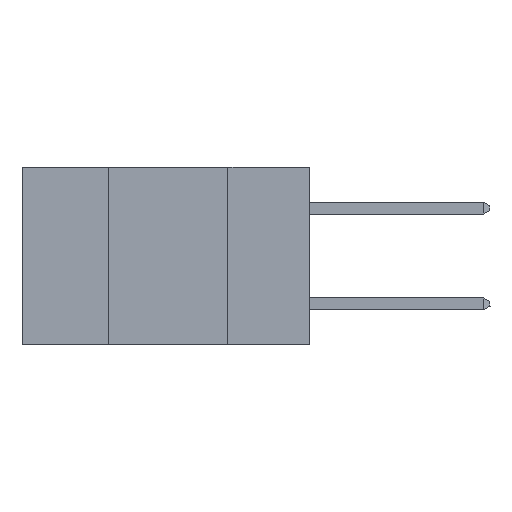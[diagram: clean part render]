
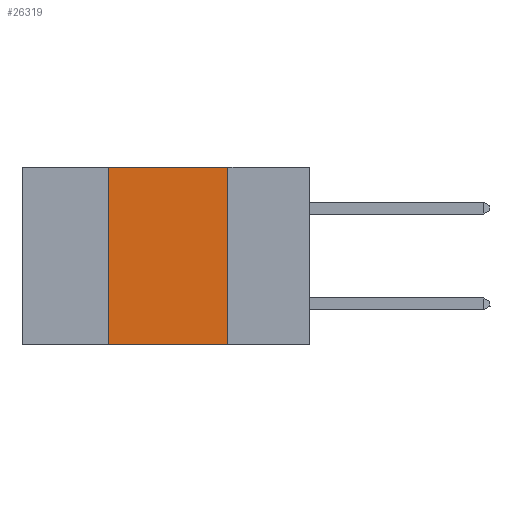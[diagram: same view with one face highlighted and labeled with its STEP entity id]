
A CAD part, left-side view. The second image highlights one B-rep face of the part: STEP entity #26319.
In plain terms, the highlighted planar face has unit normal (-1, 0, 0).
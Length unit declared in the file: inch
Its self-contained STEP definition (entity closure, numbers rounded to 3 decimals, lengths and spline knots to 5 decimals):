
#11 = CARTESIAN_POINT ( 'NONE',  ( 0., 0.6, -0.37 ) ) ;
#2732 = VERTEX_POINT ( 'NONE', #9013 ) ;
#4602 = LINE ( 'NONE', #24986, #17023 ) ;
#6655 = ORIENTED_EDGE ( 'NONE', *, *, #7911, .F. ) ;
#7911 = EDGE_CURVE ( 'NONE', #21412, #14088, #4602, .T. ) ;
#9013 = CARTESIAN_POINT ( 'NONE',  ( 0., 0.42, -0.37 ) ) ;
#9413 = PLANE ( 'NONE',  #29730 ) ;
#10476 = ORIENTED_EDGE ( 'NONE', *, *, #30962, .T. ) ;
#10655 = CARTESIAN_POINT ( 'NONE',  ( 0., 0.17, -0.37 ) ) ;
#10821 = LINE ( 'NONE', #11, #21357 ) ;
#11498 = EDGE_CURVE ( 'NONE', #2732, #21412, #20394, .T. ) ;
#11912 = DIRECTION ( 'NONE',  ( 0., 0., -1. ) ) ;
#14088 = VERTEX_POINT ( 'NONE', #14350 ) ;
#14350 = CARTESIAN_POINT ( 'NONE',  ( 0., 0.17, 0. ) ) ;
#17023 = VECTOR ( 'NONE', #19886, 39.37008 ) ;
#18873 = EDGE_LOOP ( 'NONE', ( #25091, #6655, #30802, #10476 ) ) ;
#19266 = CARTESIAN_POINT ( 'NONE',  ( 0., 0.17, 0. ) ) ;
#19292 = DIRECTION ( 'NONE',  ( 0., 0., 1. ) ) ;
#19886 = DIRECTION ( 'NONE',  ( 0., -1., 0. ) ) ;
#20394 = LINE ( 'NONE', #29831, #27486 ) ;
#21357 = VECTOR ( 'NONE', #27318, 39.37008 ) ;
#21412 = VERTEX_POINT ( 'NONE', #22739 ) ;
#22027 = DIRECTION ( 'NONE',  ( 1., 0., 0. ) ) ;
#22739 = CARTESIAN_POINT ( 'NONE',  ( 0., 0.42, 0. ) ) ;
#24282 = VERTEX_POINT ( 'NONE', #10655 ) ;
#24316 = VECTOR ( 'NONE', #27012, 39.37008 ) ;
#24408 = CARTESIAN_POINT ( 'NONE',  ( 0., 0.6, 0. ) ) ;
#24653 = EDGE_CURVE ( 'NONE', #14088, #24282, #31410, .T. ) ;
#24986 = CARTESIAN_POINT ( 'NONE',  ( 0., 0.6, 0. ) ) ;
#25091 = ORIENTED_EDGE ( 'NONE', *, *, #24653, .F. ) ;
#26319 = ADVANCED_FACE ( 'NONE', ( #28934 ), #9413, .F. ) ;
#27012 = DIRECTION ( 'NONE',  ( 0., 0., -1. ) ) ;
#27318 = DIRECTION ( 'NONE',  ( 0., -1., 0. ) ) ;
#27486 = VECTOR ( 'NONE', #19292, 39.37008 ) ;
#28934 = FACE_OUTER_BOUND ( 'NONE', #18873, .T. ) ;
#29730 = AXIS2_PLACEMENT_3D ( 'NONE', #24408, #22027, #11912 ) ;
#29831 = CARTESIAN_POINT ( 'NONE',  ( 0., 0.42, 0. ) ) ;
#30802 = ORIENTED_EDGE ( 'NONE', *, *, #11498, .F. ) ;
#30962 = EDGE_CURVE ( 'NONE', #2732, #24282, #10821, .T. ) ;
#31410 = LINE ( 'NONE', #19266, #24316 ) ;
